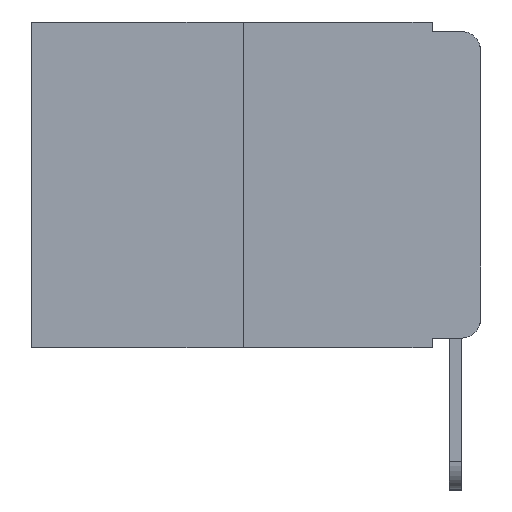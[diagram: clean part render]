
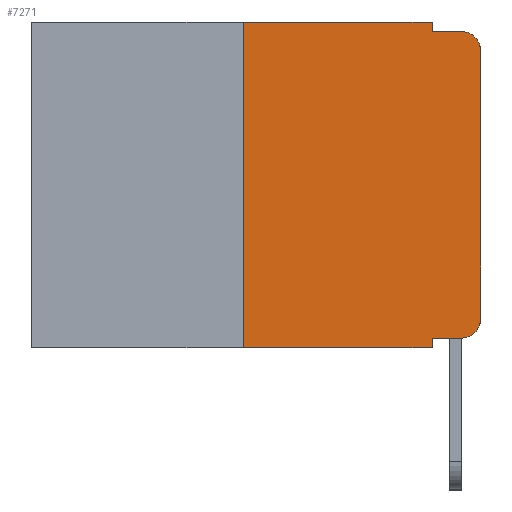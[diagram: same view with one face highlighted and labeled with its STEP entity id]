
A CAD part, left-side view. The second image highlights one B-rep face of the part: STEP entity #7271.
In plain terms, the highlighted planar face has unit normal (-1, 0, 0).
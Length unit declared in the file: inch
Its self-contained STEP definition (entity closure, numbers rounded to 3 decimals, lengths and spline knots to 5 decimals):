
#73 = ORIENTED_EDGE ( 'NONE', *, *, #6864, .T. ) ;
#186 = VERTEX_POINT ( 'NONE', #942 ) ;
#199 = DIRECTION ( 'NONE',  ( 0., 0., -1. ) ) ;
#276 = ORIENTED_EDGE ( 'NONE', *, *, #5124, .F. ) ;
#345 = VERTEX_POINT ( 'NONE', #8023 ) ;
#431 = PLANE ( 'NONE',  #5646 ) ;
#702 = EDGE_CURVE ( 'NONE', #3452, #5330, #10964, .T. ) ;
#817 = AXIS2_PLACEMENT_3D ( 'NONE', #8981, #9055, #7428 ) ;
#931 = EDGE_CURVE ( 'NONE', #7386, #9466, #1905, .T. ) ;
#942 = CARTESIAN_POINT ( 'NONE',  ( 0., 0.051, -0.343 ) ) ;
#1196 = VERTEX_POINT ( 'NONE', #10951 ) ;
#1256 = CARTESIAN_POINT ( 'NONE',  ( 0., 0., -0.313 ) ) ;
#1430 = VECTOR ( 'NONE', #4147, 39.37008 ) ;
#1485 = EDGE_CURVE ( 'NONE', #9852, #4486, #6470, .T. ) ;
#1513 = CARTESIAN_POINT ( 'NONE',  ( 0., 0.02, -0.313 ) ) ;
#1625 = VECTOR ( 'NONE', #10118, 39.37008 ) ;
#1764 = VERTEX_POINT ( 'NONE', #6718 ) ;
#1905 = LINE ( 'NONE', #10160, #4162 ) ;
#2526 = EDGE_LOOP ( 'NONE', ( #4573, #73, #4535, #276, #3783, #10665, #4677, #6329, #5786, #3362 ) ) ;
#2713 = DIRECTION ( 'NONE',  ( 0., -1., 0. ) ) ;
#3061 = AXIS2_PLACEMENT_3D ( 'NONE', #1513, #3890, #3879 ) ;
#3362 = ORIENTED_EDGE ( 'NONE', *, *, #702, .T. ) ;
#3381 = CARTESIAN_POINT ( 'NONE',  ( 0., 0.25, 0. ) ) ;
#3452 = VERTEX_POINT ( 'NONE', #7041 ) ;
#3663 = CARTESIAN_POINT ( 'NONE',  ( 0., 0.051, -0.01 ) ) ;
#3723 = DIRECTION ( 'NONE',  ( 0., -1., 0. ) ) ;
#3783 = ORIENTED_EDGE ( 'NONE', *, *, #931, .F. ) ;
#3879 = DIRECTION ( 'NONE',  ( 0., 0., -1. ) ) ;
#3890 = DIRECTION ( 'NONE',  ( -1., 0., 0. ) ) ;
#4036 = LINE ( 'NONE', #5756, #10393 ) ;
#4147 = DIRECTION ( 'NONE',  ( 0., 0., 1. ) ) ;
#4148 = VECTOR ( 'NONE', #8675, 39.37008 ) ;
#4162 = VECTOR ( 'NONE', #11021, 39.37008 ) ;
#4189 = LINE ( 'NONE', #7861, #1625 ) ;
#4486 = VERTEX_POINT ( 'NONE', #11026 ) ;
#4518 = VECTOR ( 'NONE', #3723, 39.37008 ) ;
#4535 = ORIENTED_EDGE ( 'NONE', *, *, #1485, .F. ) ;
#4573 = ORIENTED_EDGE ( 'NONE', *, *, #5450, .T. ) ;
#4677 = ORIENTED_EDGE ( 'NONE', *, *, #10415, .T. ) ;
#4794 = LINE ( 'NONE', #8501, #4518 ) ;
#5124 = EDGE_CURVE ( 'NONE', #9466, #9852, #4189, .T. ) ;
#5330 = VERTEX_POINT ( 'NONE', #1256 ) ;
#5366 = VECTOR ( 'NONE', #199, 39.37008 ) ;
#5450 = EDGE_CURVE ( 'NONE', #5330, #1764, #4036, .T. ) ;
#5646 = AXIS2_PLACEMENT_3D ( 'NONE', #10086, #10869, #10861 ) ;
#5756 = CARTESIAN_POINT ( 'NONE',  ( 0., 0., 0. ) ) ;
#5786 = ORIENTED_EDGE ( 'NONE', *, *, #10277, .T. ) ;
#6198 = DIRECTION ( 'NONE',  ( 0., 0., 1. ) ) ;
#6231 = CIRCLE ( 'NONE', #817, 0.02 ) ;
#6329 = ORIENTED_EDGE ( 'NONE', *, *, #9477, .F. ) ;
#6330 = CARTESIAN_POINT ( 'NONE',  ( 0., 0.051, 0. ) ) ;
#6470 = LINE ( 'NONE', #8218, #4148 ) ;
#6502 = CARTESIAN_POINT ( 'NONE',  ( 0., 0.25, 0. ) ) ;
#6718 = CARTESIAN_POINT ( 'NONE',  ( 0., 0., -0.03 ) ) ;
#6864 = EDGE_CURVE ( 'NONE', #1764, #4486, #6231, .T. ) ;
#7041 = CARTESIAN_POINT ( 'NONE',  ( 0., 0.02, -0.333 ) ) ;
#7176 = EDGE_CURVE ( 'NONE', #345, #7386, #10121, .T. ) ;
#7271 = ADVANCED_FACE ( 'NONE', ( #7498 ), #431, .F. ) ;
#7386 = VERTEX_POINT ( 'NONE', #6502 ) ;
#7428 = DIRECTION ( 'NONE',  ( 0., 0., -1. ) ) ;
#7498 = FACE_OUTER_BOUND ( 'NONE', #2526, .T. ) ;
#7576 = LINE ( 'NONE', #6330, #5366 ) ;
#7861 = CARTESIAN_POINT ( 'NONE',  ( 0., 0.051, 0. ) ) ;
#8023 = CARTESIAN_POINT ( 'NONE',  ( 0., 0.25, -0.343 ) ) ;
#8162 = LINE ( 'NONE', #8617, #10067 ) ;
#8218 = CARTESIAN_POINT ( 'NONE',  ( 0., 0.051, -0.01 ) ) ;
#8501 = CARTESIAN_POINT ( 'NONE',  ( 0., 0.051, -0.333 ) ) ;
#8617 = CARTESIAN_POINT ( 'NONE',  ( 0., 0.473, -0.343 ) ) ;
#8675 = DIRECTION ( 'NONE',  ( 0., -1., 0. ) ) ;
#8981 = CARTESIAN_POINT ( 'NONE',  ( 0., 0.02, -0.03 ) ) ;
#9055 = DIRECTION ( 'NONE',  ( -1., 0., 0. ) ) ;
#9466 = VERTEX_POINT ( 'NONE', #9515 ) ;
#9477 = EDGE_CURVE ( 'NONE', #1196, #186, #7576, .T. ) ;
#9515 = CARTESIAN_POINT ( 'NONE',  ( 0., 0.051, 0. ) ) ;
#9852 = VERTEX_POINT ( 'NONE', #3663 ) ;
#10067 = VECTOR ( 'NONE', #2713, 39.37008 ) ;
#10086 = CARTESIAN_POINT ( 'NONE',  ( 0., 0.473, 0. ) ) ;
#10118 = DIRECTION ( 'NONE',  ( 0., 0., -1. ) ) ;
#10121 = LINE ( 'NONE', #3381, #1430 ) ;
#10160 = CARTESIAN_POINT ( 'NONE',  ( 0., 0.473, 0. ) ) ;
#10277 = EDGE_CURVE ( 'NONE', #1196, #3452, #4794, .T. ) ;
#10393 = VECTOR ( 'NONE', #6198, 39.37008 ) ;
#10415 = EDGE_CURVE ( 'NONE', #345, #186, #8162, .T. ) ;
#10665 = ORIENTED_EDGE ( 'NONE', *, *, #7176, .F. ) ;
#10861 = DIRECTION ( 'NONE',  ( 0., 0., -1. ) ) ;
#10869 = DIRECTION ( 'NONE',  ( 1., 0., 0. ) ) ;
#10951 = CARTESIAN_POINT ( 'NONE',  ( 0., 0.051, -0.333 ) ) ;
#10964 = CIRCLE ( 'NONE', #3061, 0.02 ) ;
#11021 = DIRECTION ( 'NONE',  ( 0., -1., 0. ) ) ;
#11026 = CARTESIAN_POINT ( 'NONE',  ( 0., 0.02, -0.01 ) ) ;
